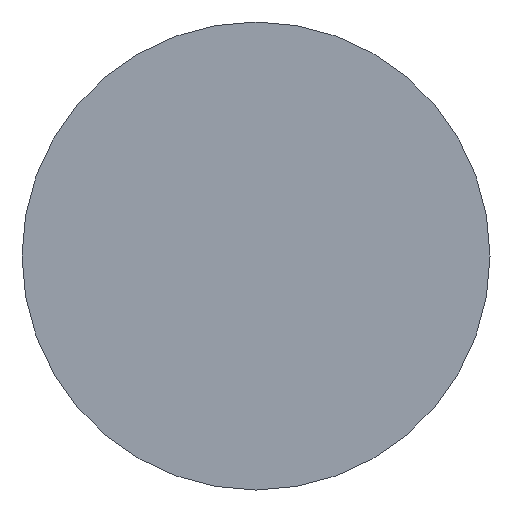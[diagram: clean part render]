
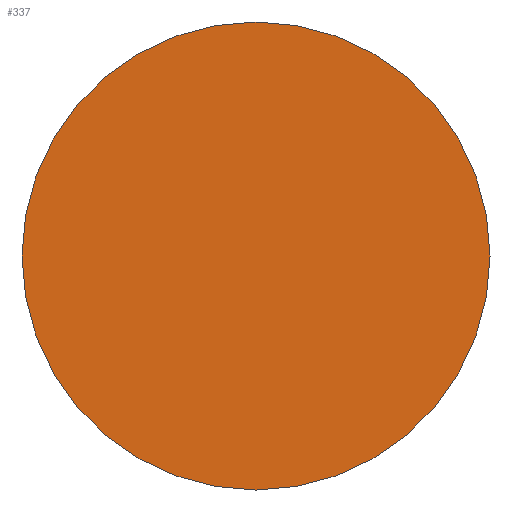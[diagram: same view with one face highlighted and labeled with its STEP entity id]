
A CAD part, front view. The second image highlights one B-rep face of the part: STEP entity #337.
In plain terms, the highlighted planar face has unit normal (0, -1, 0).
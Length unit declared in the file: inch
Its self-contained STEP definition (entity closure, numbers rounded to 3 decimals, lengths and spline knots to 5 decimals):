
#18 = DIRECTION ( 'NONE',  ( 1., 0., 0. ) ) ;
#27 = EDGE_CURVE ( 'NONE', #208, #48, #203, .T. ) ;
#34 = ORIENTED_EDGE ( 'NONE', *, *, #27, .T. ) ;
#48 = VERTEX_POINT ( 'NONE', #53 ) ;
#52 = AXIS2_PLACEMENT_3D ( 'NONE', #56, #192, #18 ) ;
#53 = CARTESIAN_POINT ( 'NONE',  ( -0.1, -0.1, 0. ) ) ;
#56 = CARTESIAN_POINT ( 'NONE',  ( 0., -0.1, 0. ) ) ;
#135 = CARTESIAN_POINT ( 'NONE',  ( 0., -0.1, 0. ) ) ;
#145 = DIRECTION ( 'NONE',  ( -1., 0., 0. ) ) ;
#147 = DIRECTION ( 'NONE',  ( 0., -1., 0. ) ) ;
#155 = CARTESIAN_POINT ( 'NONE',  ( 0., -0.1, 0. ) ) ;
#160 = PLANE ( 'NONE',  #319 ) ;
#185 = EDGE_CURVE ( 'NONE', #48, #208, #371, .T. ) ;
#192 = DIRECTION ( 'NONE',  ( 0., -1., 0. ) ) ;
#203 = CIRCLE ( 'NONE', #52, 0.1 ) ;
#208 = VERTEX_POINT ( 'NONE', #304 ) ;
#216 = DIRECTION ( 'NONE',  ( 0., -1., 0. ) ) ;
#227 = FACE_OUTER_BOUND ( 'NONE', #254, .T. ) ;
#254 = EDGE_LOOP ( 'NONE', ( #359, #34 ) ) ;
#293 = DIRECTION ( 'NONE',  ( 1., 0., 0. ) ) ;
#304 = CARTESIAN_POINT ( 'NONE',  ( 0.1, -0.1, 0. ) ) ;
#319 = AXIS2_PLACEMENT_3D ( 'NONE', #155, #147, #145 ) ;
#337 = ADVANCED_FACE ( 'NONE', ( #227 ), #160, .T. ) ;
#344 = AXIS2_PLACEMENT_3D ( 'NONE', #135, #216, #293 ) ;
#359 = ORIENTED_EDGE ( 'NONE', *, *, #185, .T. ) ;
#371 = CIRCLE ( 'NONE', #344, 0.1 ) ;
